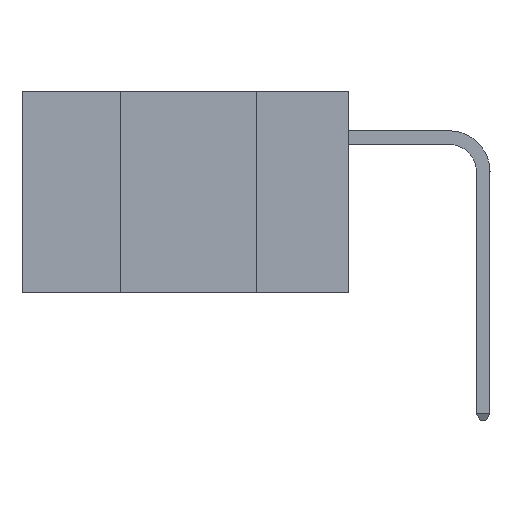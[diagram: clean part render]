
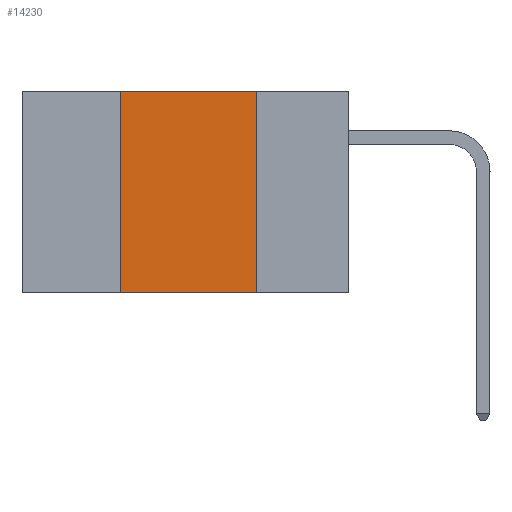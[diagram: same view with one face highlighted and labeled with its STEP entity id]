
A CAD part, left-side view. The second image highlights one B-rep face of the part: STEP entity #14230.
In plain terms, the highlighted planar face has unit normal (-1, 0, 0).
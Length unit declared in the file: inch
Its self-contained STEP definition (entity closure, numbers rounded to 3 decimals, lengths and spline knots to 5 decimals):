
#611 = EDGE_CURVE ( 'NONE', #1898, #14420, #12610, .T. ) ;
#904 = CARTESIAN_POINT ( 'NONE',  ( 0., 0.6, -0.37 ) ) ;
#1395 = ORIENTED_EDGE ( 'NONE', *, *, #14819, .F. ) ;
#1898 = VERTEX_POINT ( 'NONE', #20056 ) ;
#2083 = EDGE_CURVE ( 'NONE', #12180, #1898, #9220, .T. ) ;
#3911 = AXIS2_PLACEMENT_3D ( 'NONE', #13976, #10965, #15730 ) ;
#4332 = CARTESIAN_POINT ( 'NONE',  ( 0., 0.42, 0. ) ) ;
#4417 = LINE ( 'NONE', #11398, #4673 ) ;
#4465 = VERTEX_POINT ( 'NONE', #8347 ) ;
#4673 = VECTOR ( 'NONE', #12906, 39.37008 ) ;
#6753 = ORIENTED_EDGE ( 'NONE', *, *, #10079, .T. ) ;
#7619 = CARTESIAN_POINT ( 'NONE',  ( 0., 0.17, 0. ) ) ;
#7639 = VECTOR ( 'NONE', #12888, 39.37008 ) ;
#8331 = ORIENTED_EDGE ( 'NONE', *, *, #611, .F. ) ;
#8347 = CARTESIAN_POINT ( 'NONE',  ( 0., 0.17, -0.37 ) ) ;
#9220 = LINE ( 'NONE', #4332, #21996 ) ;
#10079 = EDGE_CURVE ( 'NONE', #12180, #4465, #16844, .T. ) ;
#10965 = DIRECTION ( 'NONE',  ( 1., 0., 0. ) ) ;
#11398 = CARTESIAN_POINT ( 'NONE',  ( 0., 0.17, 0. ) ) ;
#12180 = VERTEX_POINT ( 'NONE', #22315 ) ;
#12610 = LINE ( 'NONE', #17726, #19321 ) ;
#12888 = DIRECTION ( 'NONE',  ( 0., -1., 0. ) ) ;
#12906 = DIRECTION ( 'NONE',  ( 0., 0., -1. ) ) ;
#13976 = CARTESIAN_POINT ( 'NONE',  ( 0., 0.6, 0. ) ) ;
#14230 = ADVANCED_FACE ( 'NONE', ( #19439 ), #17697, .F. ) ;
#14420 = VERTEX_POINT ( 'NONE', #7619 ) ;
#14819 = EDGE_CURVE ( 'NONE', #14420, #4465, #4417, .T. ) ;
#15730 = DIRECTION ( 'NONE',  ( 0., 0., -1. ) ) ;
#16844 = LINE ( 'NONE', #904, #7639 ) ;
#17697 = PLANE ( 'NONE',  #3911 ) ;
#17726 = CARTESIAN_POINT ( 'NONE',  ( 0., 0.6, 0. ) ) ;
#19321 = VECTOR ( 'NONE', #21676, 39.37008 ) ;
#19439 = FACE_OUTER_BOUND ( 'NONE', #22346, .T. ) ;
#20056 = CARTESIAN_POINT ( 'NONE',  ( 0., 0.42, 0. ) ) ;
#21656 = DIRECTION ( 'NONE',  ( 0., 0., 1. ) ) ;
#21676 = DIRECTION ( 'NONE',  ( 0., -1., 0. ) ) ;
#21989 = ORIENTED_EDGE ( 'NONE', *, *, #2083, .F. ) ;
#21996 = VECTOR ( 'NONE', #21656, 39.37008 ) ;
#22315 = CARTESIAN_POINT ( 'NONE',  ( 0., 0.42, -0.37 ) ) ;
#22346 = EDGE_LOOP ( 'NONE', ( #1395, #8331, #21989, #6753 ) ) ;
